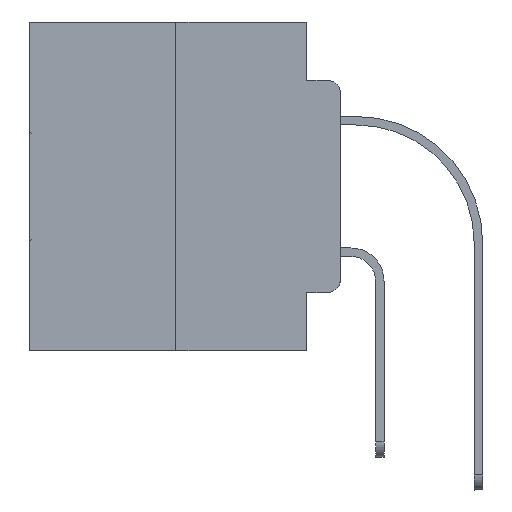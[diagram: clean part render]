
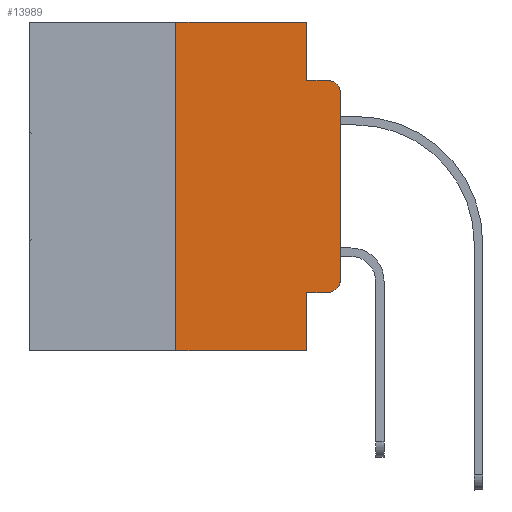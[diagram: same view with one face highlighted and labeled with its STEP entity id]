
A CAD part, left-side view. The second image highlights one B-rep face of the part: STEP entity #13989.
In plain terms, the highlighted planar face has unit normal (-1, 0, 0).
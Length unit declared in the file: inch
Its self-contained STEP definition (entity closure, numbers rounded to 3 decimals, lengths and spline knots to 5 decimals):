
#163 = VERTEX_POINT ( 'NONE', #18125 ) ;
#258 = ORIENTED_EDGE ( 'NONE', *, *, #23527, .F. ) ;
#548 = CARTESIAN_POINT ( 'NONE',  ( 0., 0., -0.3915 ) ) ;
#914 = ORIENTED_EDGE ( 'NONE', *, *, #15426, .T. ) ;
#1197 = CARTESIAN_POINT ( 'NONE',  ( 0., 0.051, 0. ) ) ;
#1221 = CARTESIAN_POINT ( 'NONE',  ( 0., 0.051, 0. ) ) ;
#1618 = EDGE_CURVE ( 'NONE', #5962, #24593, #18606, .T. ) ;
#1687 = LINE ( 'NONE', #11063, #14399 ) ;
#1702 = DIRECTION ( 'NONE',  ( 0., -1., 0. ) ) ;
#1877 = LINE ( 'NONE', #2357, #17017 ) ;
#1960 = VERTEX_POINT ( 'NONE', #20042 ) ;
#2357 = CARTESIAN_POINT ( 'NONE',  ( 0., 0.473, -0.5 ) ) ;
#2895 = AXIS2_PLACEMENT_3D ( 'NONE', #24301, #11680, #9253 ) ;
#2906 = ORIENTED_EDGE ( 'NONE', *, *, #10471, .F. ) ;
#4354 = VECTOR ( 'NONE', #26298, 39.37008 ) ;
#5229 = VERTEX_POINT ( 'NONE', #11742 ) ;
#5384 = EDGE_LOOP ( 'NONE', ( #13059, #30535, #258, #8890, #26904, #2906, #25801, #25789, #30481, #914 ) ) ;
#5962 = VERTEX_POINT ( 'NONE', #1221 ) ;
#6515 = VECTOR ( 'NONE', #21136, 39.37008 ) ;
#6832 = CARTESIAN_POINT ( 'NONE',  ( 0., 0.051, -0.0885 ) ) ;
#7752 = DIRECTION ( 'NONE',  ( 0., 0., 1. ) ) ;
#7898 = CARTESIAN_POINT ( 'NONE',  ( 0., 0.051, -0.4115 ) ) ;
#8456 = DIRECTION ( 'NONE',  ( 0., -1., 0. ) ) ;
#8890 = ORIENTED_EDGE ( 'NONE', *, *, #1618, .F. ) ;
#9253 = DIRECTION ( 'NONE',  ( 0., 0., -1. ) ) ;
#10471 = EDGE_CURVE ( 'NONE', #163, #5229, #15054, .T. ) ;
#10756 = EDGE_CURVE ( 'NONE', #24877, #17713, #28442, .T. ) ;
#11063 = CARTESIAN_POINT ( 'NONE',  ( 0., 0.051, -0.0885 ) ) ;
#11680 = DIRECTION ( 'NONE',  ( 1., 0., 0. ) ) ;
#11742 = CARTESIAN_POINT ( 'NONE',  ( 0., 0.25, 0. ) ) ;
#11904 = CARTESIAN_POINT ( 'NONE',  ( 0., 0.02, -0.3915 ) ) ;
#13059 = ORIENTED_EDGE ( 'NONE', *, *, #28914, .T. ) ;
#13989 = ADVANCED_FACE ( 'NONE', ( #17104 ), #22157, .F. ) ;
#14396 = VERTEX_POINT ( 'NONE', #19672 ) ;
#14399 = VECTOR ( 'NONE', #8456, 39.37008 ) ;
#14435 = EDGE_CURVE ( 'NONE', #5229, #5962, #16883, .T. ) ;
#14601 = LINE ( 'NONE', #24755, #26127 ) ;
#14817 = AXIS2_PLACEMENT_3D ( 'NONE', #24027, #16659, #21246 ) ;
#15054 = LINE ( 'NONE', #22581, #24126 ) ;
#15426 = EDGE_CURVE ( 'NONE', #14396, #29044, #31180, .T. ) ;
#16628 = CARTESIAN_POINT ( 'NONE',  ( 0., 0.051, 0. ) ) ;
#16659 = DIRECTION ( 'NONE',  ( -1., 0., 0. ) ) ;
#16875 = VERTEX_POINT ( 'NONE', #23257 ) ;
#16883 = LINE ( 'NONE', #21964, #28008 ) ;
#17017 = VECTOR ( 'NONE', #1702, 39.37008 ) ;
#17034 = DIRECTION ( 'NONE',  ( 0., 0., 1. ) ) ;
#17104 = FACE_OUTER_BOUND ( 'NONE', #5384, .T. ) ;
#17713 = VERTEX_POINT ( 'NONE', #28221 ) ;
#17860 = DIRECTION ( 'NONE',  ( 0., -1., 0. ) ) ;
#18125 = CARTESIAN_POINT ( 'NONE',  ( 0., 0.25, -0.5 ) ) ;
#18204 = EDGE_CURVE ( 'NONE', #16875, #14396, #20315, .T. ) ;
#18606 = LINE ( 'NONE', #16628, #4354 ) ;
#18782 = DIRECTION ( 'NONE',  ( 0., 0., -1. ) ) ;
#19672 = CARTESIAN_POINT ( 'NONE',  ( 0., 0.02, -0.4115 ) ) ;
#20042 = CARTESIAN_POINT ( 'NONE',  ( 0., 0.051, -0.5 ) ) ;
#20315 = LINE ( 'NONE', #7898, #30300 ) ;
#20981 = EDGE_CURVE ( 'NONE', #16875, #1960, #23613, .T. ) ;
#21136 = DIRECTION ( 'NONE',  ( 0., 0., -1. ) ) ;
#21246 = DIRECTION ( 'NONE',  ( 0., 0., -1. ) ) ;
#21466 = CARTESIAN_POINT ( 'NONE',  ( 0., 0., -0.1085 ) ) ;
#21887 = DIRECTION ( 'NONE',  ( -1., 0., 0. ) ) ;
#21964 = CARTESIAN_POINT ( 'NONE',  ( 0., 0.473, 0. ) ) ;
#22157 = PLANE ( 'NONE',  #2895 ) ;
#22581 = CARTESIAN_POINT ( 'NONE',  ( 0., 0.25, 0. ) ) ;
#23257 = CARTESIAN_POINT ( 'NONE',  ( 0., 0.051, -0.4115 ) ) ;
#23527 = EDGE_CURVE ( 'NONE', #24593, #17713, #1687, .T. ) ;
#23613 = LINE ( 'NONE', #1197, #6515 ) ;
#24027 = CARTESIAN_POINT ( 'NONE',  ( 0., 0.02, -0.1085 ) ) ;
#24126 = VECTOR ( 'NONE', #17034, 39.37008 ) ;
#24301 = CARTESIAN_POINT ( 'NONE',  ( 0., 0.473, 0. ) ) ;
#24593 = VERTEX_POINT ( 'NONE', #6832 ) ;
#24755 = CARTESIAN_POINT ( 'NONE',  ( 0., 0., 0. ) ) ;
#24877 = VERTEX_POINT ( 'NONE', #21466 ) ;
#25789 = ORIENTED_EDGE ( 'NONE', *, *, #20981, .F. ) ;
#25801 = ORIENTED_EDGE ( 'NONE', *, *, #32026, .T. ) ;
#26127 = VECTOR ( 'NONE', #7752, 39.37008 ) ;
#26298 = DIRECTION ( 'NONE',  ( 0., 0., -1. ) ) ;
#26573 = DIRECTION ( 'NONE',  ( 0., -1., 0. ) ) ;
#26904 = ORIENTED_EDGE ( 'NONE', *, *, #14435, .F. ) ;
#28008 = VECTOR ( 'NONE', #26573, 39.37008 ) ;
#28221 = CARTESIAN_POINT ( 'NONE',  ( 0., 0.02, -0.0885 ) ) ;
#28442 = CIRCLE ( 'NONE', #14817, 0.02 ) ;
#28914 = EDGE_CURVE ( 'NONE', #29044, #24877, #14601, .T. ) ;
#29044 = VERTEX_POINT ( 'NONE', #548 ) ;
#29616 = AXIS2_PLACEMENT_3D ( 'NONE', #11904, #21887, #18782 ) ;
#30300 = VECTOR ( 'NONE', #17860, 39.37008 ) ;
#30481 = ORIENTED_EDGE ( 'NONE', *, *, #18204, .T. ) ;
#30535 = ORIENTED_EDGE ( 'NONE', *, *, #10756, .T. ) ;
#31180 = CIRCLE ( 'NONE', #29616, 0.02 ) ;
#32026 = EDGE_CURVE ( 'NONE', #163, #1960, #1877, .T. ) ;
